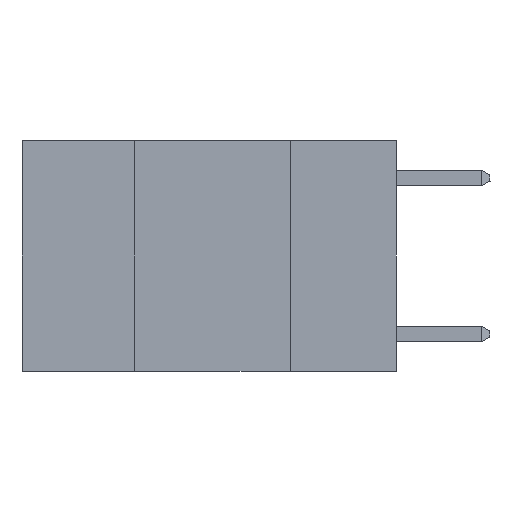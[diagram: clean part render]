
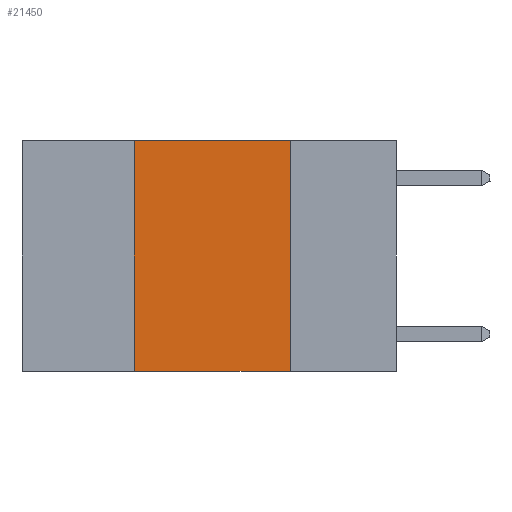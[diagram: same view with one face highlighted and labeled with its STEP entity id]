
A CAD part, left-side view. The second image highlights one B-rep face of the part: STEP entity #21450.
In plain terms, the highlighted planar face has unit normal (-1, 0, 0).
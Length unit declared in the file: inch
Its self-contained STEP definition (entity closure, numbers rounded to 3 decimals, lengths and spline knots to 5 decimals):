
#400 = DIRECTION ( 'NONE',  ( 0., 0., 1. ) ) ;
#467 = VERTEX_POINT ( 'NONE', #6067 ) ;
#1703 = VERTEX_POINT ( 'NONE', #20929 ) ;
#1824 = CARTESIAN_POINT ( 'NONE',  ( 0., 0.6, 0. ) ) ;
#3721 = CARTESIAN_POINT ( 'NONE',  ( 0., 0.6, -0.37 ) ) ;
#4864 = ORIENTED_EDGE ( 'NONE', *, *, #21253, .F. ) ;
#4882 = CARTESIAN_POINT ( 'NONE',  ( 0., 0.17, 0. ) ) ;
#4937 = EDGE_CURVE ( 'NONE', #467, #1703, #16829, .T. ) ;
#5548 = AXIS2_PLACEMENT_3D ( 'NONE', #1824, #7701, #20915 ) ;
#5707 = DIRECTION ( 'NONE',  ( 0., -1., 0. ) ) ;
#6067 = CARTESIAN_POINT ( 'NONE',  ( 0., 0.42, -0.37 ) ) ;
#6095 = CARTESIAN_POINT ( 'NONE',  ( 0., 0.6, 0. ) ) ;
#6101 = VECTOR ( 'NONE', #5707, 39.37008 ) ;
#7612 = PLANE ( 'NONE',  #5548 ) ;
#7701 = DIRECTION ( 'NONE',  ( 1., 0., 0. ) ) ;
#9038 = DIRECTION ( 'NONE',  ( 0., -1., 0. ) ) ;
#9782 = LINE ( 'NONE', #19580, #14198 ) ;
#10163 = ORIENTED_EDGE ( 'NONE', *, *, #14313, .F. ) ;
#12814 = DIRECTION ( 'NONE',  ( 0., 0., -1. ) ) ;
#13782 = VECTOR ( 'NONE', #9038, 39.37008 ) ;
#14198 = VECTOR ( 'NONE', #400, 39.37008 ) ;
#14313 = EDGE_CURVE ( 'NONE', #15378, #1703, #17470, .T. ) ;
#15201 = VERTEX_POINT ( 'NONE', #18975 ) ;
#15378 = VERTEX_POINT ( 'NONE', #4882 ) ;
#16829 = LINE ( 'NONE', #3721, #6101 ) ;
#17470 = LINE ( 'NONE', #24042, #18039 ) ;
#17596 = ORIENTED_EDGE ( 'NONE', *, *, #20116, .F. ) ;
#18039 = VECTOR ( 'NONE', #12814, 39.37008 ) ;
#18832 = LINE ( 'NONE', #6095, #13782 ) ;
#18975 = CARTESIAN_POINT ( 'NONE',  ( 0., 0.42, 0. ) ) ;
#19580 = CARTESIAN_POINT ( 'NONE',  ( 0., 0.42, 0. ) ) ;
#20105 = ORIENTED_EDGE ( 'NONE', *, *, #4937, .T. ) ;
#20116 = EDGE_CURVE ( 'NONE', #467, #15201, #9782, .T. ) ;
#20915 = DIRECTION ( 'NONE',  ( 0., 0., -1. ) ) ;
#20929 = CARTESIAN_POINT ( 'NONE',  ( 0., 0.17, -0.37 ) ) ;
#21253 = EDGE_CURVE ( 'NONE', #15201, #15378, #18832, .T. ) ;
#21450 = ADVANCED_FACE ( 'NONE', ( #24007 ), #7612, .F. ) ;
#23091 = EDGE_LOOP ( 'NONE', ( #10163, #4864, #17596, #20105 ) ) ;
#24007 = FACE_OUTER_BOUND ( 'NONE', #23091, .T. ) ;
#24042 = CARTESIAN_POINT ( 'NONE',  ( 0., 0.17, 0. ) ) ;
